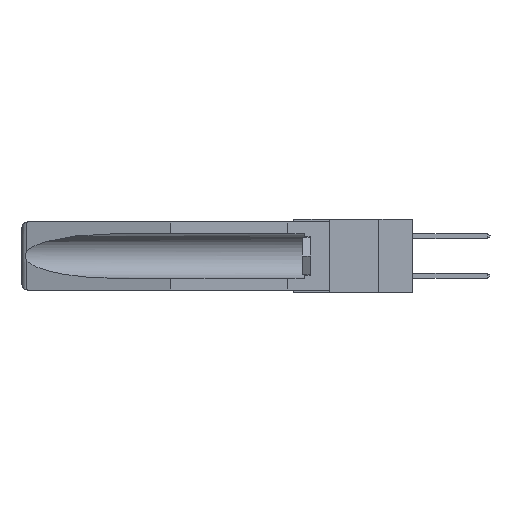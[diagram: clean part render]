
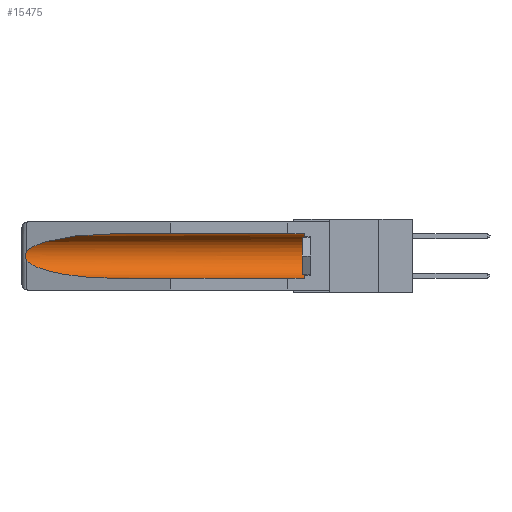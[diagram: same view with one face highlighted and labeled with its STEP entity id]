
A CAD part, left-side view. The second image highlights one B-rep face of the part: STEP entity #15475.
In plain terms, the highlighted cylindrical face has radius 2.857 mm (diameter 5.715 mm), a partial arc.
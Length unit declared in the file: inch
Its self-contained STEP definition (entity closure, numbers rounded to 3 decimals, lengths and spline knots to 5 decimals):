
#47 = CARTESIAN_POINT ( 'NONE',  ( 0.155, -0.30754, -0.284 ) ) ;
#78 = CARTESIAN_POINT ( 'NONE',  ( 0.26537, 1.52718, -0.19328 ) ) ;
#251 = CARTESIAN_POINT ( 'NONE',  ( 0.2673, 1.5327, -0.16383 ) ) ;
#1403 = CARTESIAN_POINT ( 'NONE',  ( 0.25451, 1.48313, -0.24835 ) ) ;
#1480 = ORIENTED_EDGE ( 'NONE', *, *, #3825, .T. ) ;
#1509 = VERTEX_POINT ( 'NONE', #15399 ) ;
#1935 = VECTOR ( 'NONE', #7806, 39.37008 ) ;
#2231 = CARTESIAN_POINT ( 'NONE',  ( 0.2675, 1.53308, -0.17534 ) ) ;
#3023 = CARTESIAN_POINT ( 'NONE',  ( 0.155, 0.126, -0.1715 ) ) ;
#3079 = LINE ( 'NONE', #47, #5885 ) ;
#3492 = CARTESIAN_POINT ( 'NONE',  ( 0.155, 1.07973, -0.284 ) ) ;
#3825 = EDGE_CURVE ( 'NONE', #18140, #11763, #10370, .T. ) ;
#3918 = CARTESIAN_POINT ( 'NONE',  ( 0.26654, 1.53092, -0.15636 ) ) ;
#4827 =( BOUNDED_CURVE ( )  B_SPLINE_CURVE ( 3, ( #22058, #5706, #21884, #23920 ),
 .UNSPECIFIED., .F., .F. ) 
 B_SPLINE_CURVE_WITH_KNOTS ( ( 4, 4 ),
 ( 4.71239, 6.08839 ),
 .UNSPECIFIED. ) 
 CURVE ( )  GEOMETRIC_REPRESENTATION_ITEM ( )  RATIONAL_B_SPLINE_CURVE ( ( 1., 0.848, 0.848, 1. ) ) 
 REPRESENTATION_ITEM ( '' )  );
#5407 = EDGE_CURVE ( 'NONE', #10528, #18140, #12643, .T. ) ;
#5706 = CARTESIAN_POINT ( 'NONE',  ( 0.21114, 1.30732, -0.059 ) ) ;
#5775 = CARTESIAN_POINT ( 'NONE',  ( 0.26537, 1.52718, -0.19328 ) ) ;
#5822 = CARTESIAN_POINT ( 'NONE',  ( 0.26537, 1.52718, -0.14972 ) ) ;
#5885 = VECTOR ( 'NONE', #12476, 39.37008 ) ;
#5951 = EDGE_CURVE ( 'NONE', #23691, #10528, #4827, .T. ) ;
#5971 = ORIENTED_EDGE ( 'NONE', *, *, #5407, .T. ) ;
#6295 = CARTESIAN_POINT ( 'NONE',  ( 0.26597, 1.5296, -0.19026 ) ) ;
#6600 = FACE_OUTER_BOUND ( 'NONE', #16509, .T. ) ;
#7197 = ORIENTED_EDGE ( 'NONE', *, *, #7254, .T. ) ;
#7254 = EDGE_CURVE ( 'NONE', #1509, #23691, #18929, .T. ) ;
#7806 = DIRECTION ( 'NONE',  ( 0., 1., 0. ) ) ;
#7880 = CARTESIAN_POINT ( 'NONE',  ( 0.155, 1.07973, -0.284 ) ) ;
#8289 = ORIENTED_EDGE ( 'NONE', *, *, #19347, .T. ) ;
#8420 = DIRECTION ( 'NONE',  ( 0., -1., 0. ) ) ;
#9254 = DIRECTION ( 'NONE',  ( 0., 1., 0. ) ) ;
#9327 = AXIS2_PLACEMENT_3D ( 'NONE', #3023, #8420, #12401 ) ;
#10052 = EDGE_CURVE ( 'NONE', #24057, #11763, #3079, .T. ) ;
#10370 =( BOUNDED_CURVE ( )  B_SPLINE_CURVE ( 3, ( #23869, #1403, #15553, #3492 ),
 .UNSPECIFIED., .F., .F. ) 
 B_SPLINE_CURVE_WITH_KNOTS ( ( 4, 4 ),
 ( 0.1948, 1.5708 ),
 .UNSPECIFIED. ) 
 CURVE ( )  GEOMETRIC_REPRESENTATION_ITEM ( )  RATIONAL_B_SPLINE_CURVE ( ( 1., 0.848, 0.848, 1. ) ) 
 REPRESENTATION_ITEM ( '' )  );
#10528 = VERTEX_POINT ( 'NONE', #19436 ) ;
#11763 = VERTEX_POINT ( 'NONE', #7880 ) ;
#12401 = DIRECTION ( 'NONE',  ( 0., 0., 1. ) ) ;
#12476 = DIRECTION ( 'NONE',  ( 0., 1., 0. ) ) ;
#12643 = B_SPLINE_CURVE_WITH_KNOTS ( 'NONE', 3,
 ( #5822, #13655, #3918, #251, #14344, #2231, #18339, #22429, #6295, #78 ),
 .UNSPECIFIED., .F., .F.,
 ( 4, 2, 2, 2, 4 ),
 ( 0., 0.00029, 0.00058, 0.00087, 0.00117 ),
 .UNSPECIFIED. ) ;
#12754 = CIRCLE ( 'NONE', #9327, 0.1125 ) ;
#13655 = CARTESIAN_POINT ( 'NONE',  ( 0.26597, 1.52961, -0.15275 ) ) ;
#14344 = CARTESIAN_POINT ( 'NONE',  ( 0.2675, 1.53308, -0.16763 ) ) ;
#14398 = DIRECTION ( 'NONE',  ( 0., 0., 1. ) ) ;
#14504 = CYLINDRICAL_SURFACE ( 'NONE', #25836, 0.1125 ) ;
#15399 = CARTESIAN_POINT ( 'NONE',  ( 0.155, 0.126, -0.059 ) ) ;
#15475 = ADVANCED_FACE ( 'NONE', ( #6600 ), #14504, .F. ) ;
#15553 = CARTESIAN_POINT ( 'NONE',  ( 0.21114, 1.30732, -0.284 ) ) ;
#15580 = ORIENTED_EDGE ( 'NONE', *, *, #5951, .T. ) ;
#15678 = CARTESIAN_POINT ( 'NONE',  ( 0.155, -0.30754, -0.059 ) ) ;
#16509 = EDGE_LOOP ( 'NONE', ( #15580, #5971, #1480, #19520, #8289, #7197 ) ) ;
#17829 = CARTESIAN_POINT ( 'NONE',  ( 0.155, 1.07973, -0.059 ) ) ;
#18140 = VERTEX_POINT ( 'NONE', #5775 ) ;
#18339 = CARTESIAN_POINT ( 'NONE',  ( 0.2673, 1.53269, -0.17917 ) ) ;
#18929 = LINE ( 'NONE', #15678, #1935 ) ;
#19347 = EDGE_CURVE ( 'NONE', #24057, #1509, #12754, .T. ) ;
#19436 = CARTESIAN_POINT ( 'NONE',  ( 0.26537, 1.52718, -0.14972 ) ) ;
#19520 = ORIENTED_EDGE ( 'NONE', *, *, #10052, .F. ) ;
#21884 = CARTESIAN_POINT ( 'NONE',  ( 0.25451, 1.48313, -0.09465 ) ) ;
#22058 = CARTESIAN_POINT ( 'NONE',  ( 0.155, 1.07973, -0.059 ) ) ;
#22429 = CARTESIAN_POINT ( 'NONE',  ( 0.26655, 1.53094, -0.18657 ) ) ;
#22944 = CARTESIAN_POINT ( 'NONE',  ( 0.155, 0.126, -0.284 ) ) ;
#23691 = VERTEX_POINT ( 'NONE', #17829 ) ;
#23869 = CARTESIAN_POINT ( 'NONE',  ( 0.26537, 1.52718, -0.19328 ) ) ;
#23920 = CARTESIAN_POINT ( 'NONE',  ( 0.26537, 1.52718, -0.14972 ) ) ;
#24057 = VERTEX_POINT ( 'NONE', #22944 ) ;
#25324 = CARTESIAN_POINT ( 'NONE',  ( 0.155, -0.30754, -0.1715 ) ) ;
#25836 = AXIS2_PLACEMENT_3D ( 'NONE', #25324, #9254, #14398 ) ;
